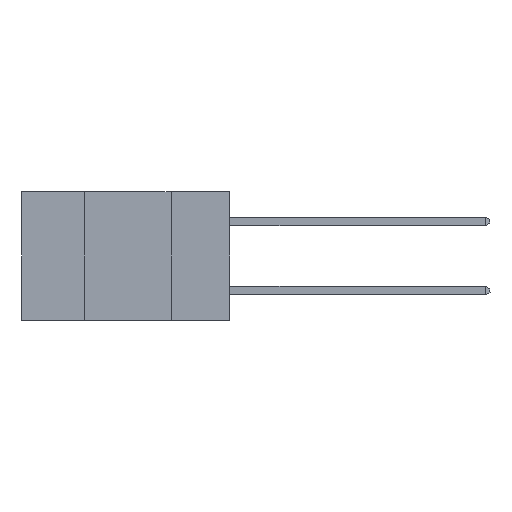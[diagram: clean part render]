
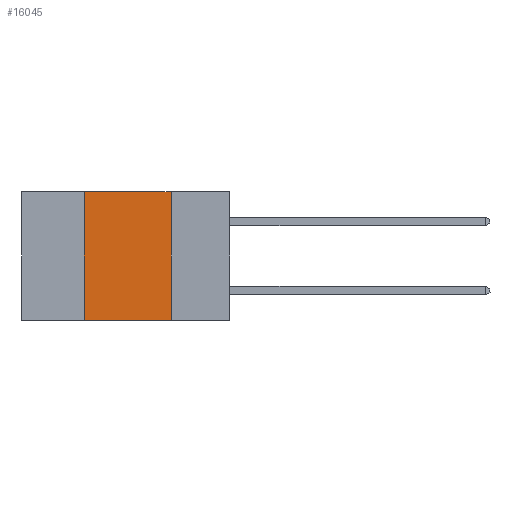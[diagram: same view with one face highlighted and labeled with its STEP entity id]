
A CAD part, left-side view. The second image highlights one B-rep face of the part: STEP entity #16045.
In plain terms, the highlighted planar face has unit normal (-1, 0, 0).
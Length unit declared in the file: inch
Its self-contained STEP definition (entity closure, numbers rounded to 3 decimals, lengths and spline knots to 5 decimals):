
#107 = CARTESIAN_POINT ( 'NONE',  ( 0., 0.42, -0.37 ) ) ;
#1327 = ORIENTED_EDGE ( 'NONE', *, *, #10732, .F. ) ;
#1379 = CARTESIAN_POINT ( 'NONE',  ( 0., 0.6, 0. ) ) ;
#2729 = EDGE_CURVE ( 'NONE', #8534, #8448, #15670, .T. ) ;
#3679 = ORIENTED_EDGE ( 'NONE', *, *, #12287, .T. ) ;
#4038 = DIRECTION ( 'NONE',  ( 0., 0., -1. ) ) ;
#4062 = CARTESIAN_POINT ( 'NONE',  ( 0., 0.17, 0. ) ) ;
#4210 = PLANE ( 'NONE',  #15509 ) ;
#4709 = DIRECTION ( 'NONE',  ( 0., 0., -1. ) ) ;
#5273 = VECTOR ( 'NONE', #11612, 39.37008 ) ;
#5659 = LINE ( 'NONE', #12553, #12369 ) ;
#7937 = DIRECTION ( 'NONE',  ( 1., 0., 0. ) ) ;
#8166 = LINE ( 'NONE', #15601, #5273 ) ;
#8365 = DIRECTION ( 'NONE',  ( 0., 0., 1. ) ) ;
#8448 = VERTEX_POINT ( 'NONE', #16768 ) ;
#8534 = VERTEX_POINT ( 'NONE', #107 ) ;
#9911 = EDGE_CURVE ( 'NONE', #15324, #14155, #5659, .T. ) ;
#10081 = ORIENTED_EDGE ( 'NONE', *, *, #2729, .F. ) ;
#10132 = FACE_OUTER_BOUND ( 'NONE', #13039, .T. ) ;
#10425 = ORIENTED_EDGE ( 'NONE', *, *, #9911, .F. ) ;
#10732 = EDGE_CURVE ( 'NONE', #8448, #15324, #14575, .T. ) ;
#10766 = VECTOR ( 'NONE', #8365, 39.37008 ) ;
#11460 = CARTESIAN_POINT ( 'NONE',  ( 0., 0.17, -0.37 ) ) ;
#11612 = DIRECTION ( 'NONE',  ( 0., -1., 0. ) ) ;
#11766 = CARTESIAN_POINT ( 'NONE',  ( 0., 0.6, 0. ) ) ;
#12287 = EDGE_CURVE ( 'NONE', #8534, #14155, #8166, .T. ) ;
#12369 = VECTOR ( 'NONE', #4709, 39.37008 ) ;
#12553 = CARTESIAN_POINT ( 'NONE',  ( 0., 0.17, 0. ) ) ;
#13039 = EDGE_LOOP ( 'NONE', ( #10425, #1327, #10081, #3679 ) ) ;
#13481 = CARTESIAN_POINT ( 'NONE',  ( 0., 0.42, 0. ) ) ;
#14124 = VECTOR ( 'NONE', #15825, 39.37008 ) ;
#14155 = VERTEX_POINT ( 'NONE', #11460 ) ;
#14575 = LINE ( 'NONE', #11766, #14124 ) ;
#15324 = VERTEX_POINT ( 'NONE', #4062 ) ;
#15509 = AXIS2_PLACEMENT_3D ( 'NONE', #1379, #7937, #4038 ) ;
#15601 = CARTESIAN_POINT ( 'NONE',  ( 0., 0.6, -0.37 ) ) ;
#15670 = LINE ( 'NONE', #13481, #10766 ) ;
#15825 = DIRECTION ( 'NONE',  ( 0., -1., 0. ) ) ;
#16045 = ADVANCED_FACE ( 'NONE', ( #10132 ), #4210, .F. ) ;
#16768 = CARTESIAN_POINT ( 'NONE',  ( 0., 0.42, 0. ) ) ;
